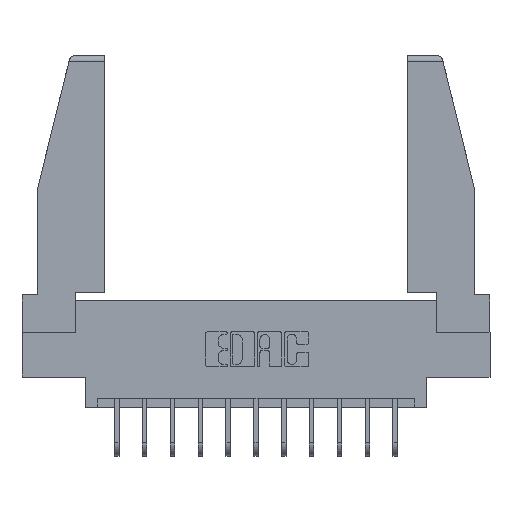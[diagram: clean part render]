
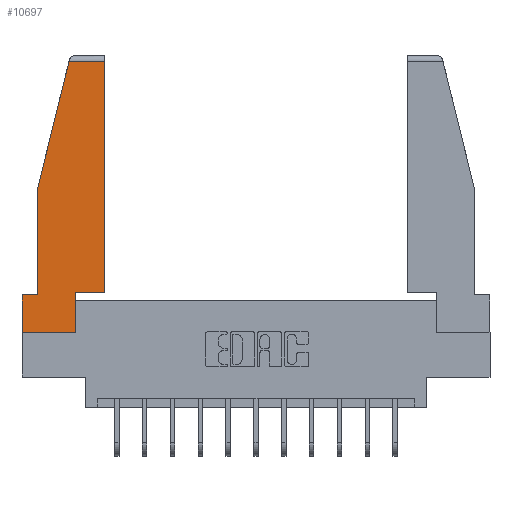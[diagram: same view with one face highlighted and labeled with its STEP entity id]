
A CAD part, top view. The second image highlights one B-rep face of the part: STEP entity #10697.
In plain terms, the highlighted planar face has unit normal (0, 0, 1).
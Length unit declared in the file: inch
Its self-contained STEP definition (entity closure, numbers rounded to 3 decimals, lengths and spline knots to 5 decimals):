
#184 = CARTESIAN_POINT ( 'NONE',  ( 0.297, 0.223, 0. ) ) ;
#190 = CARTESIAN_POINT ( 'NONE',  ( 0.461, 1.52, 0. ) ) ;
#432 = ORIENTED_EDGE ( 'NONE', *, *, #14520, .T. ) ;
#541 = CARTESIAN_POINT ( 'NONE',  ( 0.086, 0.8, 0. ) ) ;
#750 = ORIENTED_EDGE ( 'NONE', *, *, #9221, .T. ) ;
#1016 = CARTESIAN_POINT ( 'NONE',  ( 0.2636, 1.52, 0. ) ) ;
#1089 = EDGE_CURVE ( 'NONE', #10422, #14129, #3651, .T. ) ;
#1217 = VECTOR ( 'NONE', #11637, 39.37008 ) ;
#1298 = VECTOR ( 'NONE', #7854, 39.37008 ) ;
#1449 = VERTEX_POINT ( 'NONE', #190 ) ;
#1617 = VECTOR ( 'NONE', #13189, 39.37008 ) ;
#1737 = LINE ( 'NONE', #16758, #14763 ) ;
#2033 = LINE ( 'NONE', #2806, #1617 ) ;
#2060 = VERTEX_POINT ( 'NONE', #14544 ) ;
#2315 = CARTESIAN_POINT ( 'NONE',  ( 0.086, 0.21, 0. ) ) ;
#2806 = CARTESIAN_POINT ( 'NONE',  ( 0.086, 0.8, 0. ) ) ;
#2842 = DIRECTION ( 'NONE',  ( 0., -1., 0. ) ) ;
#2844 = DIRECTION ( 'NONE',  ( -1., 0., 0. ) ) ;
#3372 = LINE ( 'NONE', #9172, #5204 ) ;
#3651 = LINE ( 'NONE', #184, #13837 ) ;
#4106 = CARTESIAN_POINT ( 'NONE',  ( 0., 0.21, 0. ) ) ;
#4258 = EDGE_CURVE ( 'NONE', #7772, #12407, #3372, .T. ) ;
#4423 = PLANE ( 'NONE',  #12615 ) ;
#4460 = EDGE_CURVE ( 'NONE', #7507, #12426, #2033, .T. ) ;
#4543 = FACE_OUTER_BOUND ( 'NONE', #16240, .T. ) ;
#4794 = LINE ( 'NONE', #9226, #1298 ) ;
#5204 = VECTOR ( 'NONE', #2842, 39.37008 ) ;
#5693 = EDGE_CURVE ( 'NONE', #12426, #7772, #6941, .T. ) ;
#6324 = ORIENTED_EDGE ( 'NONE', *, *, #5693, .T. ) ;
#6455 = VECTOR ( 'NONE', #2844, 39.37008 ) ;
#6941 = LINE ( 'NONE', #4106, #9814 ) ;
#6987 = CARTESIAN_POINT ( 'NONE',  ( 0.461, 0.223, 0. ) ) ;
#7154 = LINE ( 'NONE', #15628, #1217 ) ;
#7507 = VERTEX_POINT ( 'NONE', #541 ) ;
#7772 = VERTEX_POINT ( 'NONE', #7860 ) ;
#7851 = LINE ( 'NONE', #16664, #16001 ) ;
#7854 = DIRECTION ( 'NONE',  ( 0., 1., 0. ) ) ;
#7860 = CARTESIAN_POINT ( 'NONE',  ( 0., 0.21, 0. ) ) ;
#7922 = CARTESIAN_POINT ( 'NONE',  ( 0., 0., 0. ) ) ;
#8231 = CARTESIAN_POINT ( 'NONE',  ( 0., 0., 0. ) ) ;
#9099 = LINE ( 'NONE', #12051, #6455 ) ;
#9172 = CARTESIAN_POINT ( 'NONE',  ( 0., 0.21, 0. ) ) ;
#9221 = EDGE_CURVE ( 'NONE', #2060, #10422, #1737, .T. ) ;
#9226 = CARTESIAN_POINT ( 'NONE',  ( 0.461, 0.223, 0. ) ) ;
#9561 = EDGE_CURVE ( 'NONE', #14129, #1449, #4794, .T. ) ;
#9814 = VECTOR ( 'NONE', #11937, 39.37008 ) ;
#10194 = DIRECTION ( 'NONE',  ( 0., 1., 0. ) ) ;
#10422 = VERTEX_POINT ( 'NONE', #11360 ) ;
#10697 = ADVANCED_FACE ( 'NONE', ( #4543 ), #4423, .T. ) ;
#11143 = DIRECTION ( 'NONE',  ( 0., 0., 1. ) ) ;
#11316 = EDGE_CURVE ( 'NONE', #14297, #7507, #7154, .T. ) ;
#11360 = CARTESIAN_POINT ( 'NONE',  ( 0.297, 0.223, 0. ) ) ;
#11455 = ORIENTED_EDGE ( 'NONE', *, *, #4258, .T. ) ;
#11637 = DIRECTION ( 'NONE',  ( -0.239, -0.971, 0. ) ) ;
#11644 = ORIENTED_EDGE ( 'NONE', *, *, #11316, .T. ) ;
#11937 = DIRECTION ( 'NONE',  ( -1., 0., 0. ) ) ;
#11938 = DIRECTION ( 'NONE',  ( 1., 0., 0. ) ) ;
#11990 = ORIENTED_EDGE ( 'NONE', *, *, #1089, .T. ) ;
#12051 = CARTESIAN_POINT ( 'NONE',  ( 0., 1.52, 0. ) ) ;
#12148 = ORIENTED_EDGE ( 'NONE', *, *, #15155, .T. ) ;
#12337 = ORIENTED_EDGE ( 'NONE', *, *, #4460, .T. ) ;
#12406 = ORIENTED_EDGE ( 'NONE', *, *, #9561, .T. ) ;
#12407 = VERTEX_POINT ( 'NONE', #8231 ) ;
#12426 = VERTEX_POINT ( 'NONE', #2315 ) ;
#12615 = AXIS2_PLACEMENT_3D ( 'NONE', #7922, #11143, #15108 ) ;
#12749 = DIRECTION ( 'NONE',  ( 1., 0., 0. ) ) ;
#13189 = DIRECTION ( 'NONE',  ( 0., -1., 0. ) ) ;
#13837 = VECTOR ( 'NONE', #11938, 39.37008 ) ;
#14129 = VERTEX_POINT ( 'NONE', #6987 ) ;
#14297 = VERTEX_POINT ( 'NONE', #1016 ) ;
#14520 = EDGE_CURVE ( 'NONE', #1449, #14297, #9099, .T. ) ;
#14544 = CARTESIAN_POINT ( 'NONE',  ( 0.297, 0., 0. ) ) ;
#14763 = VECTOR ( 'NONE', #10194, 39.37008 ) ;
#15108 = DIRECTION ( 'NONE',  ( 1., 0., 0. ) ) ;
#15155 = EDGE_CURVE ( 'NONE', #12407, #2060, #7851, .T. ) ;
#15628 = CARTESIAN_POINT ( 'NONE',  ( 0.271, 1.55, 0. ) ) ;
#16001 = VECTOR ( 'NONE', #12749, 39.37008 ) ;
#16240 = EDGE_LOOP ( 'NONE', ( #12406, #432, #11644, #12337, #6324, #11455, #12148, #750, #11990 ) ) ;
#16664 = CARTESIAN_POINT ( 'NONE',  ( 0., 0., 0. ) ) ;
#16758 = CARTESIAN_POINT ( 'NONE',  ( 0.297, 0., 0. ) ) ;
